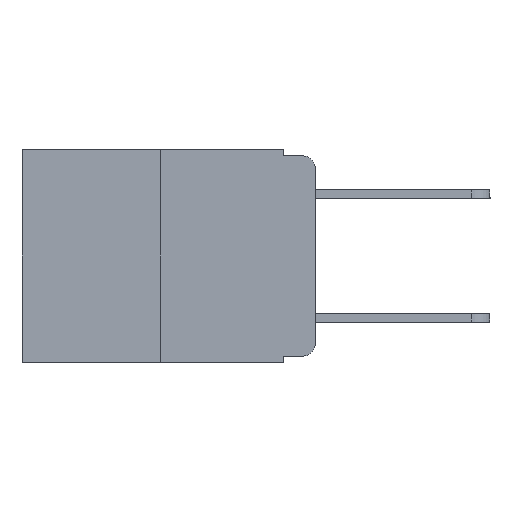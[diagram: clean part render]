
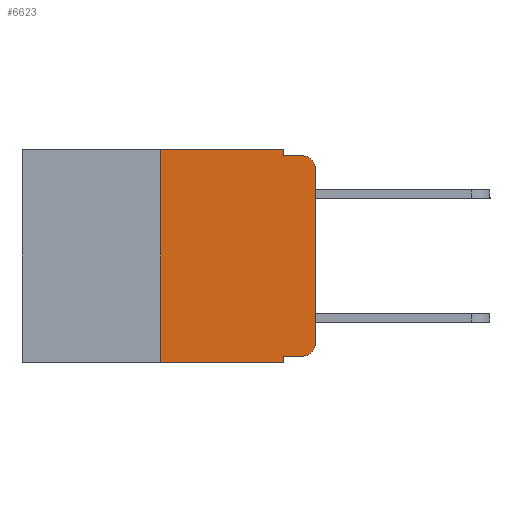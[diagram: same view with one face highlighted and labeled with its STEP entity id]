
A CAD part, left-side view. The second image highlights one B-rep face of the part: STEP entity #6623.
In plain terms, the highlighted planar face has unit normal (-1, 0, 0).
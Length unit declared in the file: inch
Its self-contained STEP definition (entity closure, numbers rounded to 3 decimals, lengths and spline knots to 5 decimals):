
#135 = CARTESIAN_POINT ( 'NONE',  ( 0., 0.25, -0.343 ) ) ;
#437 = EDGE_CURVE ( 'NONE', #3346, #14419, #19110, .T. ) ;
#742 = VERTEX_POINT ( 'NONE', #1705 ) ;
#768 = ORIENTED_EDGE ( 'NONE', *, *, #7210, .F. ) ;
#853 = LINE ( 'NONE', #1791, #4871 ) ;
#1185 = VERTEX_POINT ( 'NONE', #4609 ) ;
#1346 = EDGE_CURVE ( 'NONE', #742, #3346, #14804, .T. ) ;
#1531 = VECTOR ( 'NONE', #11851, 39.37008 ) ;
#1705 = CARTESIAN_POINT ( 'NONE',  ( 0., 0.25, 0. ) ) ;
#1791 = CARTESIAN_POINT ( 'NONE',  ( 0., 0.473, -0.343 ) ) ;
#2164 = ORIENTED_EDGE ( 'NONE', *, *, #9032, .T. ) ;
#2445 = LINE ( 'NONE', #3691, #10933 ) ;
#2458 = VERTEX_POINT ( 'NONE', #17907 ) ;
#2918 = ORIENTED_EDGE ( 'NONE', *, *, #19052, .F. ) ;
#3243 = CARTESIAN_POINT ( 'NONE',  ( 0., 0., -0.03 ) ) ;
#3346 = VERTEX_POINT ( 'NONE', #15547 ) ;
#3514 = DIRECTION ( 'NONE',  ( 0., -1., 0. ) ) ;
#3647 = CARTESIAN_POINT ( 'NONE',  ( 0., 0.02, -0.03 ) ) ;
#3691 = CARTESIAN_POINT ( 'NONE',  ( 0., 0.051, -0.333 ) ) ;
#4466 = DIRECTION ( 'NONE',  ( 0., -1., 0. ) ) ;
#4609 = CARTESIAN_POINT ( 'NONE',  ( 0., 0.051, -0.333 ) ) ;
#4626 = VERTEX_POINT ( 'NONE', #17004 ) ;
#4659 = VERTEX_POINT ( 'NONE', #17655 ) ;
#4871 = VECTOR ( 'NONE', #3514, 39.37008 ) ;
#4891 = PLANE ( 'NONE',  #17526 ) ;
#5060 = EDGE_CURVE ( 'NONE', #1185, #10481, #6056, .T. ) ;
#5318 = DIRECTION ( 'NONE',  ( 0., 0., -1. ) ) ;
#5852 = DIRECTION ( 'NONE',  ( 0., 0., 1. ) ) ;
#6046 = VECTOR ( 'NONE', #11977, 39.37008 ) ;
#6056 = LINE ( 'NONE', #15888, #1531 ) ;
#6567 = DIRECTION ( 'NONE',  ( 0., 0., -1. ) ) ;
#6623 = ADVANCED_FACE ( 'NONE', ( #16122 ), #4891, .F. ) ;
#7210 = EDGE_CURVE ( 'NONE', #13159, #742, #16106, .T. ) ;
#7220 = VECTOR ( 'NONE', #5852, 39.37008 ) ;
#7349 = ORIENTED_EDGE ( 'NONE', *, *, #9103, .T. ) ;
#7753 = CARTESIAN_POINT ( 'NONE',  ( 0., 0.25, 0. ) ) ;
#8189 = CIRCLE ( 'NONE', #10804, 0.02 ) ;
#8287 = VERTEX_POINT ( 'NONE', #3243 ) ;
#8923 = CARTESIAN_POINT ( 'NONE',  ( 0., 0.02, -0.313 ) ) ;
#9032 = EDGE_CURVE ( 'NONE', #13159, #10481, #853, .T. ) ;
#9103 = EDGE_CURVE ( 'NONE', #8287, #4626, #8189, .T. ) ;
#9504 = ORIENTED_EDGE ( 'NONE', *, *, #14684, .T. ) ;
#9580 = AXIS2_PLACEMENT_3D ( 'NONE', #8923, #18474, #10415 ) ;
#10114 = EDGE_LOOP ( 'NONE', ( #9504, #7349, #2918, #10581, #10992, #768, #2164, #11866, #11215, #10867 ) ) ;
#10185 = LINE ( 'NONE', #17251, #6046 ) ;
#10247 = CARTESIAN_POINT ( 'NONE',  ( 0., 0.051, -0.343 ) ) ;
#10415 = DIRECTION ( 'NONE',  ( 0., 0., -1. ) ) ;
#10481 = VERTEX_POINT ( 'NONE', #10247 ) ;
#10581 = ORIENTED_EDGE ( 'NONE', *, *, #437, .F. ) ;
#10804 = AXIS2_PLACEMENT_3D ( 'NONE', #3647, #14182, #5318 ) ;
#10867 = ORIENTED_EDGE ( 'NONE', *, *, #11469, .T. ) ;
#10933 = VECTOR ( 'NONE', #18216, 39.37008 ) ;
#10992 = ORIENTED_EDGE ( 'NONE', *, *, #1346, .F. ) ;
#11174 = CARTESIAN_POINT ( 'NONE',  ( 0., 0.051, -0.01 ) ) ;
#11206 = LINE ( 'NONE', #15973, #7220 ) ;
#11215 = ORIENTED_EDGE ( 'NONE', *, *, #17506, .T. ) ;
#11469 = EDGE_CURVE ( 'NONE', #2458, #4659, #12406, .T. ) ;
#11683 = CARTESIAN_POINT ( 'NONE',  ( 0., 0.473, 0. ) ) ;
#11851 = DIRECTION ( 'NONE',  ( 0., 0., -1. ) ) ;
#11866 = ORIENTED_EDGE ( 'NONE', *, *, #5060, .F. ) ;
#11977 = DIRECTION ( 'NONE',  ( 0., -1., 0. ) ) ;
#12406 = CIRCLE ( 'NONE', #9580, 0.02 ) ;
#13159 = VERTEX_POINT ( 'NONE', #135 ) ;
#13424 = DIRECTION ( 'NONE',  ( 0., 0., -1. ) ) ;
#13842 = CARTESIAN_POINT ( 'NONE',  ( 0., 0.473, 0. ) ) ;
#14182 = DIRECTION ( 'NONE',  ( -1., 0., 0. ) ) ;
#14390 = VECTOR ( 'NONE', #4466, 39.37008 ) ;
#14419 = VERTEX_POINT ( 'NONE', #11174 ) ;
#14684 = EDGE_CURVE ( 'NONE', #4659, #8287, #11206, .T. ) ;
#14804 = LINE ( 'NONE', #11683, #14390 ) ;
#15201 = DIRECTION ( 'NONE',  ( 1., 0., 0. ) ) ;
#15547 = CARTESIAN_POINT ( 'NONE',  ( 0., 0.051, 0. ) ) ;
#15679 = VECTOR ( 'NONE', #13424, 39.37008 ) ;
#15711 = VECTOR ( 'NONE', #18792, 39.37008 ) ;
#15888 = CARTESIAN_POINT ( 'NONE',  ( 0., 0.051, 0. ) ) ;
#15973 = CARTESIAN_POINT ( 'NONE',  ( 0., 0., 0. ) ) ;
#16106 = LINE ( 'NONE', #7753, #15711 ) ;
#16122 = FACE_OUTER_BOUND ( 'NONE', #10114, .T. ) ;
#17004 = CARTESIAN_POINT ( 'NONE',  ( 0., 0.02, -0.01 ) ) ;
#17251 = CARTESIAN_POINT ( 'NONE',  ( 0., 0.051, -0.01 ) ) ;
#17506 = EDGE_CURVE ( 'NONE', #1185, #2458, #2445, .T. ) ;
#17526 = AXIS2_PLACEMENT_3D ( 'NONE', #13842, #15201, #6567 ) ;
#17655 = CARTESIAN_POINT ( 'NONE',  ( 0., 0., -0.313 ) ) ;
#17907 = CARTESIAN_POINT ( 'NONE',  ( 0., 0.02, -0.333 ) ) ;
#18216 = DIRECTION ( 'NONE',  ( 0., -1., 0. ) ) ;
#18474 = DIRECTION ( 'NONE',  ( -1., 0., 0. ) ) ;
#18792 = DIRECTION ( 'NONE',  ( 0., 0., 1. ) ) ;
#19052 = EDGE_CURVE ( 'NONE', #14419, #4626, #10185, .T. ) ;
#19110 = LINE ( 'NONE', #19276, #15679 ) ;
#19276 = CARTESIAN_POINT ( 'NONE',  ( 0., 0.051, 0. ) ) ;
